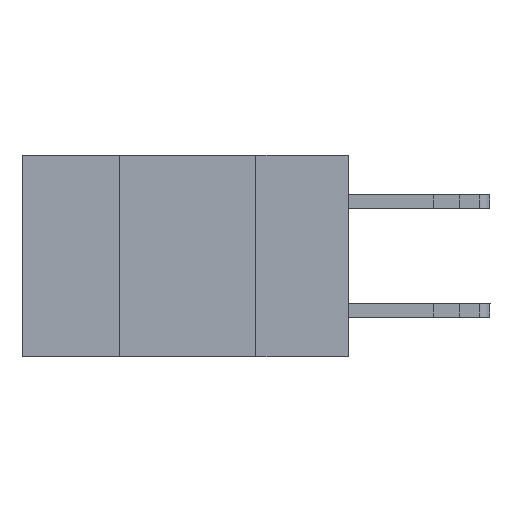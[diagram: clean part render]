
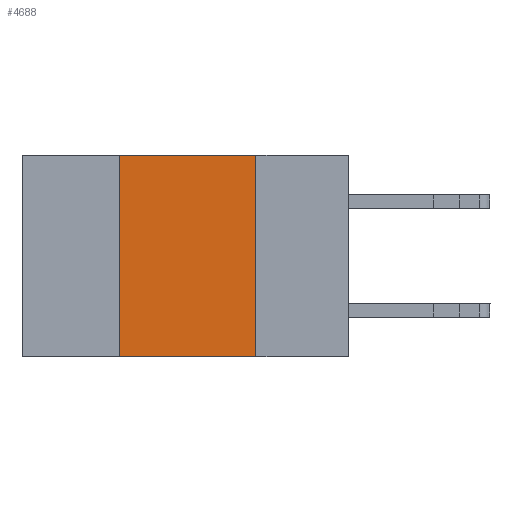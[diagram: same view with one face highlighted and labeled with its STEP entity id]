
A CAD part, left-side view. The second image highlights one B-rep face of the part: STEP entity #4688.
In plain terms, the highlighted planar face has unit normal (-1, 0, 0).
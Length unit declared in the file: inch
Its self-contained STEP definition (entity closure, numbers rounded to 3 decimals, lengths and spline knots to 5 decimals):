
#572 = LINE ( 'NONE', #8210, #7126 ) ;
#1048 = LINE ( 'NONE', #5783, #19295 ) ;
#1146 = CARTESIAN_POINT ( 'NONE',  ( 0., 0.6, 0. ) ) ;
#1707 = DIRECTION ( 'NONE',  ( 1., 0., 0. ) ) ;
#2697 = LINE ( 'NONE', #18059, #11893 ) ;
#2923 = DIRECTION ( 'NONE',  ( 0., -1., 0. ) ) ;
#3773 = EDGE_CURVE ( 'NONE', #9957, #9281, #2697, .T. ) ;
#4049 = ORIENTED_EDGE ( 'NONE', *, *, #3773, .T. ) ;
#4321 = AXIS2_PLACEMENT_3D ( 'NONE', #12048, #1707, #13789 ) ;
#4688 = ADVANCED_FACE ( 'NONE', ( #7268 ), #5120, .F. ) ;
#5120 = PLANE ( 'NONE',  #4321 ) ;
#5783 = CARTESIAN_POINT ( 'NONE',  ( 0., 0.42, -0.37 ) ) ;
#5920 = ORIENTED_EDGE ( 'NONE', *, *, #10849, .F. ) ;
#6005 = CARTESIAN_POINT ( 'NONE',  ( 0., 0.42, -0.37 ) ) ;
#6127 = DIRECTION ( 'NONE',  ( 0., -1., 0. ) ) ;
#7001 = ORIENTED_EDGE ( 'NONE', *, *, #9074, .F. ) ;
#7068 = VERTEX_POINT ( 'NONE', #14901 ) ;
#7126 = VECTOR ( 'NONE', #9945, 39.37008 ) ;
#7268 = FACE_OUTER_BOUND ( 'NONE', #17396, .T. ) ;
#8210 = CARTESIAN_POINT ( 'NONE',  ( 0., 0.17, -0.37 ) ) ;
#9074 = EDGE_CURVE ( 'NONE', #13914, #7068, #18399, .T. ) ;
#9281 = VERTEX_POINT ( 'NONE', #10985 ) ;
#9332 = VECTOR ( 'NONE', #2923, 39.37008 ) ;
#9945 = DIRECTION ( 'NONE',  ( 0., 0., -1. ) ) ;
#9957 = VERTEX_POINT ( 'NONE', #6005 ) ;
#10849 = EDGE_CURVE ( 'NONE', #7068, #9281, #572, .T. ) ;
#10985 = CARTESIAN_POINT ( 'NONE',  ( 0., 0.17, -0.37 ) ) ;
#11893 = VECTOR ( 'NONE', #6127, 39.37008 ) ;
#12048 = CARTESIAN_POINT ( 'NONE',  ( 0., 0.6, 0. ) ) ;
#12641 = ORIENTED_EDGE ( 'NONE', *, *, #20644, .F. ) ;
#12683 = DIRECTION ( 'NONE',  ( 0., 0., 1. ) ) ;
#13789 = DIRECTION ( 'NONE',  ( 0., 0., -1. ) ) ;
#13914 = VERTEX_POINT ( 'NONE', #21798 ) ;
#14901 = CARTESIAN_POINT ( 'NONE',  ( 0., 0.17, 0. ) ) ;
#17396 = EDGE_LOOP ( 'NONE', ( #5920, #7001, #12641, #4049 ) ) ;
#18059 = CARTESIAN_POINT ( 'NONE',  ( 0., 0.6, -0.37 ) ) ;
#18399 = LINE ( 'NONE', #1146, #9332 ) ;
#19295 = VECTOR ( 'NONE', #12683, 39.37008 ) ;
#20644 = EDGE_CURVE ( 'NONE', #9957, #13914, #1048, .T. ) ;
#21798 = CARTESIAN_POINT ( 'NONE',  ( 0., 0.42, 0. ) ) ;
